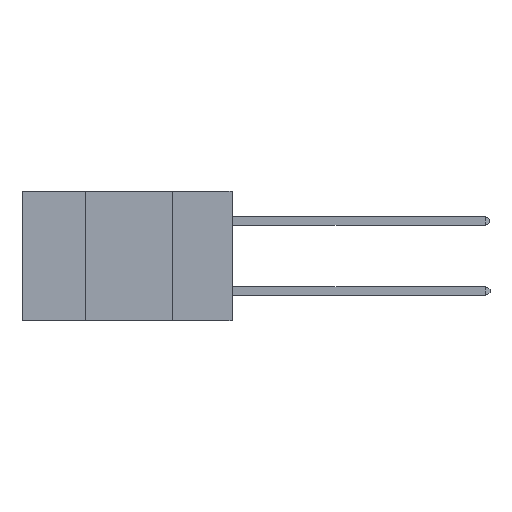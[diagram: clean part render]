
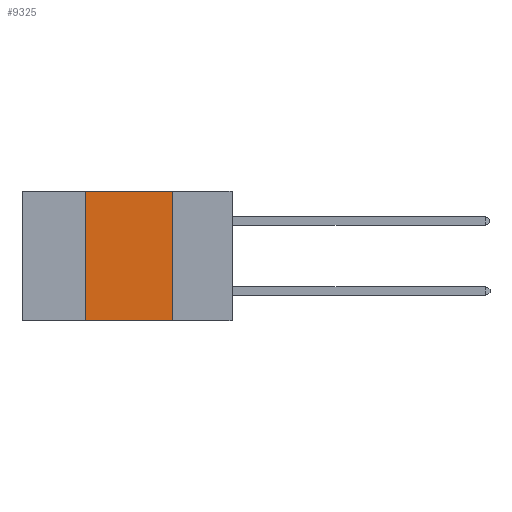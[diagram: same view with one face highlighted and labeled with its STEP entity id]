
A CAD part, left-side view. The second image highlights one B-rep face of the part: STEP entity #9325.
In plain terms, the highlighted planar face has unit normal (-1, 0, 0).
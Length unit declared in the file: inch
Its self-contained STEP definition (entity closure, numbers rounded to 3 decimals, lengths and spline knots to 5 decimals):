
#967 = PLANE ( 'NONE',  #15975 ) ;
#1240 = VECTOR ( 'NONE', #7886, 39.37008 ) ;
#1462 = EDGE_CURVE ( 'NONE', #4963, #9677, #11858, .T. ) ;
#2651 = EDGE_CURVE ( 'NONE', #4963, #13467, #12013, .T. ) ;
#3420 = VECTOR ( 'NONE', #9266, 39.37008 ) ;
#4963 = VERTEX_POINT ( 'NONE', #6611 ) ;
#5185 = DIRECTION ( 'NONE',  ( 0., 0., -1. ) ) ;
#6140 = CARTESIAN_POINT ( 'NONE',  ( 0., 0.6, 0. ) ) ;
#6507 = ORIENTED_EDGE ( 'NONE', *, *, #1462, .T. ) ;
#6611 = CARTESIAN_POINT ( 'NONE',  ( 0., 0.42, -0.37 ) ) ;
#7555 = VECTOR ( 'NONE', #17534, 39.37008 ) ;
#7857 = DIRECTION ( 'NONE',  ( 0., 0., -1. ) ) ;
#7886 = DIRECTION ( 'NONE',  ( 0., -1., 0. ) ) ;
#7898 = ORIENTED_EDGE ( 'NONE', *, *, #10217, .F. ) ;
#7968 = EDGE_LOOP ( 'NONE', ( #7898, #21699, #12128, #6507 ) ) ;
#8192 = FACE_OUTER_BOUND ( 'NONE', #7968, .T. ) ;
#8665 = LINE ( 'NONE', #13435, #21318 ) ;
#9266 = DIRECTION ( 'NONE',  ( 0., -1., 0. ) ) ;
#9325 = ADVANCED_FACE ( 'NONE', ( #8192 ), #967, .F. ) ;
#9677 = VERTEX_POINT ( 'NONE', #20041 ) ;
#10217 = EDGE_CURVE ( 'NONE', #20265, #9677, #8665, .T. ) ;
#10784 = CARTESIAN_POINT ( 'NONE',  ( 0., 0.6, -0.37 ) ) ;
#11858 = LINE ( 'NONE', #10784, #3420 ) ;
#12013 = LINE ( 'NONE', #18511, #7555 ) ;
#12128 = ORIENTED_EDGE ( 'NONE', *, *, #2651, .F. ) ;
#13435 = CARTESIAN_POINT ( 'NONE',  ( 0., 0.17, 0. ) ) ;
#13467 = VERTEX_POINT ( 'NONE', #16353 ) ;
#14626 = LINE ( 'NONE', #17783, #1240 ) ;
#15892 = CARTESIAN_POINT ( 'NONE',  ( 0., 0.17, 0. ) ) ;
#15975 = AXIS2_PLACEMENT_3D ( 'NONE', #6140, #17754, #7857 ) ;
#16353 = CARTESIAN_POINT ( 'NONE',  ( 0., 0.42, 0. ) ) ;
#17534 = DIRECTION ( 'NONE',  ( 0., 0., 1. ) ) ;
#17754 = DIRECTION ( 'NONE',  ( 1., 0., 0. ) ) ;
#17783 = CARTESIAN_POINT ( 'NONE',  ( 0., 0.6, 0. ) ) ;
#18511 = CARTESIAN_POINT ( 'NONE',  ( 0., 0.42, 0. ) ) ;
#18557 = EDGE_CURVE ( 'NONE', #13467, #20265, #14626, .T. ) ;
#20041 = CARTESIAN_POINT ( 'NONE',  ( 0., 0.17, -0.37 ) ) ;
#20265 = VERTEX_POINT ( 'NONE', #15892 ) ;
#21318 = VECTOR ( 'NONE', #5185, 39.37008 ) ;
#21699 = ORIENTED_EDGE ( 'NONE', *, *, #18557, .F. ) ;
